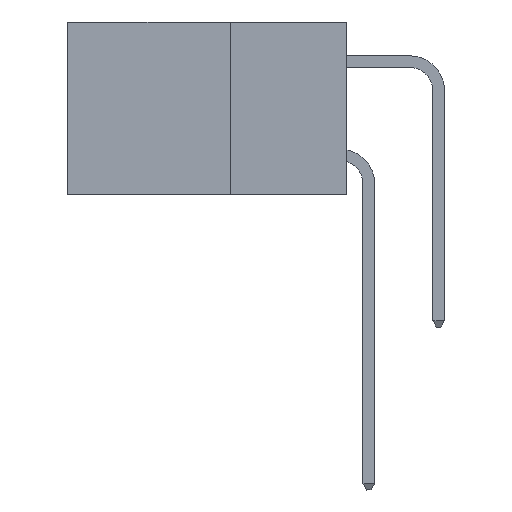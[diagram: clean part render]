
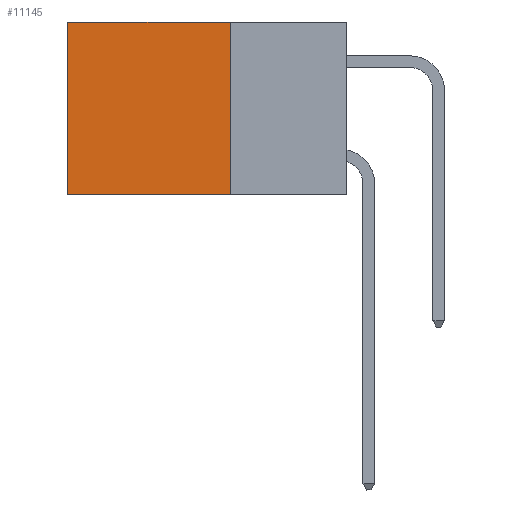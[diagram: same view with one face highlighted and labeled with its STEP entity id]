
A CAD part, left-side view. The second image highlights one B-rep face of the part: STEP entity #11145.
In plain terms, the highlighted planar face has unit normal (-1, 0, 0).
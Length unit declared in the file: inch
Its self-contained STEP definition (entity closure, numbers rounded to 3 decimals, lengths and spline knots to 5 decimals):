
#2331 = EDGE_CURVE ( 'NONE', #3072, #12530, #24698, .T. ) ;
#2481 = CARTESIAN_POINT ( 'NONE',  ( 0.2875, 0.25, 0. ) ) ;
#3072 = VERTEX_POINT ( 'NONE', #7596 ) ;
#3287 = CARTESIAN_POINT ( 'NONE',  ( 0.2875, 0.25, 0. ) ) ;
#4618 = CARTESIAN_POINT ( 'NONE',  ( 0.2875, 0.6, 0. ) ) ;
#5858 = VERTEX_POINT ( 'NONE', #4618 ) ;
#7596 = CARTESIAN_POINT ( 'NONE',  ( 0.2875, 0.25, -0.37 ) ) ;
#8025 = DIRECTION ( 'NONE',  ( 1., 0., 0. ) ) ;
#10809 = ORIENTED_EDGE ( 'NONE', *, *, #16899, .T. ) ;
#11145 = ADVANCED_FACE ( 'NONE', ( #26898 ), #14874, .F. ) ;
#11772 = DIRECTION ( 'NONE',  ( 0., 0., -1. ) ) ;
#12530 = VERTEX_POINT ( 'NONE', #27511 ) ;
#12613 = LINE ( 'NONE', #3287, #35837 ) ;
#13078 = AXIS2_PLACEMENT_3D ( 'NONE', #20660, #8025, #11772 ) ;
#14874 = PLANE ( 'NONE',  #13078 ) ;
#14990 = DIRECTION ( 'NONE',  ( 0., 1., 0. ) ) ;
#15103 = ORIENTED_EDGE ( 'NONE', *, *, #24209, .F. ) ;
#16135 = DIRECTION ( 'NONE',  ( 0., 1., 0. ) ) ;
#16899 = EDGE_CURVE ( 'NONE', #34234, #5858, #12613, .T. ) ;
#17599 = EDGE_LOOP ( 'NONE', ( #22008, #40265, #15103, #10809 ) ) ;
#19397 = DIRECTION ( 'NONE',  ( 0., 0., -1. ) ) ;
#19611 = LINE ( 'NONE', #35747, #34179 ) ;
#20660 = CARTESIAN_POINT ( 'NONE',  ( 0.2875, 0.25, 0. ) ) ;
#20789 = CARTESIAN_POINT ( 'NONE',  ( 0.2875, 0.25, -0.37 ) ) ;
#21531 = LINE ( 'NONE', #2481, #35419 ) ;
#21685 = VECTOR ( 'NONE', #14990, 39.37008 ) ;
#22008 = ORIENTED_EDGE ( 'NONE', *, *, #33575, .T. ) ;
#24209 = EDGE_CURVE ( 'NONE', #34234, #3072, #21531, .T. ) ;
#24698 = LINE ( 'NONE', #20789, #21685 ) ;
#26898 = FACE_OUTER_BOUND ( 'NONE', #17599, .T. ) ;
#27511 = CARTESIAN_POINT ( 'NONE',  ( 0.2875, 0.6, -0.37 ) ) ;
#33189 = CARTESIAN_POINT ( 'NONE',  ( 0.2875, 0.25, 0. ) ) ;
#33575 = EDGE_CURVE ( 'NONE', #5858, #12530, #19611, .T. ) ;
#34156 = DIRECTION ( 'NONE',  ( 0., 0., -1. ) ) ;
#34179 = VECTOR ( 'NONE', #19397, 39.37008 ) ;
#34234 = VERTEX_POINT ( 'NONE', #33189 ) ;
#35419 = VECTOR ( 'NONE', #34156, 39.37008 ) ;
#35747 = CARTESIAN_POINT ( 'NONE',  ( 0.2875, 0.6, 0. ) ) ;
#35837 = VECTOR ( 'NONE', #16135, 39.37008 ) ;
#40265 = ORIENTED_EDGE ( 'NONE', *, *, #2331, .F. ) ;
